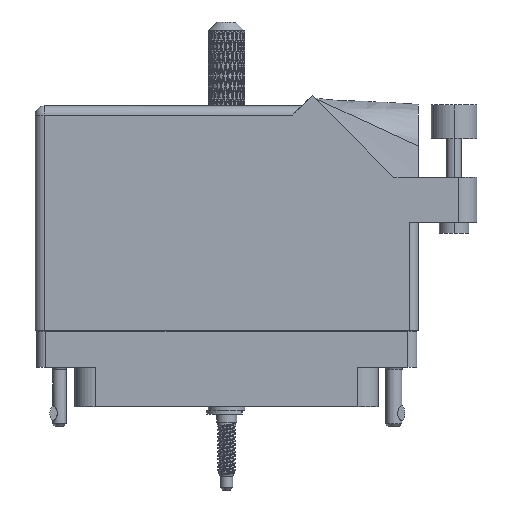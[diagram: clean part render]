
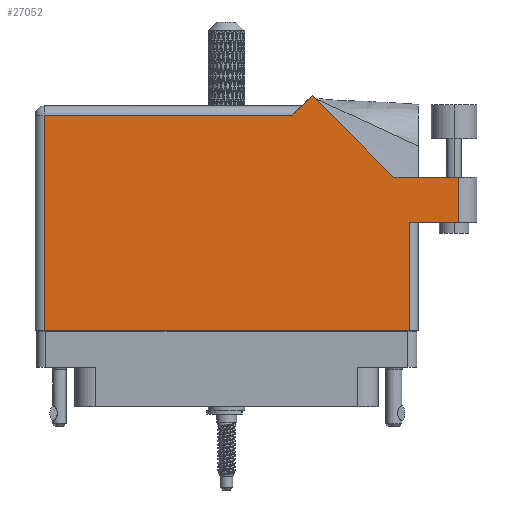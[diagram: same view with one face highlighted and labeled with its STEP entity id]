
A CAD part, front view. The second image highlights one B-rep face of the part: STEP entity #27052.
In plain terms, the highlighted face is planar.
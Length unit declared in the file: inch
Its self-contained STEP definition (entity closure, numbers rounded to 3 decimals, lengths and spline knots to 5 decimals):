
#1107 = CARTESIAN_POINT ( 'NONE',  ( 1.706, 0.944, 0.455 ) ) ;
#1807 = LINE ( 'NONE', #1107, #78496 ) ;
#3629 = VERTEX_POINT ( 'NONE', #45650 ) ;
#8971 = CARTESIAN_POINT ( 'NONE',  ( -1.244, -0.1, 0.455 ) ) ;
#10130 = DIRECTION ( 'NONE',  ( 1., 0., 0. ) ) ;
#15489 = PLANE ( 'NONE',  #107749 ) ;
#17531 = CARTESIAN_POINT ( 'NONE',  ( 1.14042, 0.944, 0.455 ) ) ;
#17821 = VERTEX_POINT ( 'NONE', #45904 ) ;
#18321 = VERTEX_POINT ( 'NONE', #92838 ) ;
#19076 = CARTESIAN_POINT ( 'NONE',  ( 0.513, 1.43, 0.455 ) ) ;
#19303 = CARTESIAN_POINT ( 'NONE',  ( -1.244, -0.1, 0.455 ) ) ;
#20014 = ORIENTED_EDGE ( 'NONE', *, *, #60571, .T. ) ;
#25834 = VECTOR ( 'NONE', #10130, 39.37008 ) ;
#27052 = ADVANCED_FACE ( 'NONE', ( #53091 ), #15489, .F. ) ;
#29794 = LINE ( 'NONE', #17531, #75566 ) ;
#30705 = VECTOR ( 'NONE', #89515, 39.37008 ) ;
#34439 = CARTESIAN_POINT ( 'NONE',  ( -1.306, 1.43, 0.455 ) ) ;
#35619 = CARTESIAN_POINT ( 'NONE',  ( 1.581, 0.944, 0.455 ) ) ;
#37146 = VERTEX_POINT ( 'NONE', #19303 ) ;
#37289 = DIRECTION ( 'NONE',  ( 1., 0., 0. ) ) ;
#37291 = DIRECTION ( 'NONE',  ( -0.707, 0.707, 0. ) ) ;
#38185 = ORIENTED_EDGE ( 'NONE', *, *, #101634, .T. ) ;
#40395 = CARTESIAN_POINT ( 'NONE',  ( 1.244, 0.637, 0.455 ) ) ;
#41104 = ORIENTED_EDGE ( 'NONE', *, *, #90923, .T. ) ;
#44049 = CARTESIAN_POINT ( 'NONE',  ( 1.581, 0.637, 0.455 ) ) ;
#45650 = CARTESIAN_POINT ( 'NONE',  ( 0.58371, 1.50071, 0.455 ) ) ;
#45701 = ORIENTED_EDGE ( 'NONE', *, *, #86420, .T. ) ;
#45733 = VECTOR ( 'NONE', #76660, 39.37008 ) ;
#45904 = CARTESIAN_POINT ( 'NONE',  ( 1.244, 0.637, 0.455 ) ) ;
#47489 = DIRECTION ( 'NONE',  ( -0.707, -0.707, 0. ) ) ;
#48413 = VECTOR ( 'NONE', #47489, 39.37008 ) ;
#49285 = VERTEX_POINT ( 'NONE', #35619 ) ;
#50863 = LINE ( 'NONE', #113680, #25834 ) ;
#53091 = FACE_OUTER_BOUND ( 'NONE', #87425, .T. ) ;
#54775 = CARTESIAN_POINT ( 'NONE',  ( 1.14042, 0.944, 0.455 ) ) ;
#56794 = LINE ( 'NONE', #81420, #117391 ) ;
#60571 = EDGE_CURVE ( 'NONE', #18321, #94752, #56794, .T. ) ;
#63276 = DIRECTION ( 'NONE',  ( -1., 0., 0. ) ) ;
#63346 = EDGE_CURVE ( 'NONE', #49285, #69453, #1807, .T. ) ;
#67115 = DIRECTION ( 'NONE',  ( -1., 0., 0. ) ) ;
#69453 = VERTEX_POINT ( 'NONE', #54775 ) ;
#70926 = LINE ( 'NONE', #111983, #112257 ) ;
#71590 = EDGE_CURVE ( 'NONE', #37146, #112481, #70926, .T. ) ;
#75566 = VECTOR ( 'NONE', #37291, 39.37008 ) ;
#76660 = DIRECTION ( 'NONE',  ( 0., 1., 0. ) ) ;
#76928 = CARTESIAN_POINT ( 'NONE',  ( -1.244, 1.368, 0.455 ) ) ;
#78496 = VECTOR ( 'NONE', #67115, 39.37008 ) ;
#79142 = ORIENTED_EDGE ( 'NONE', *, *, #71590, .T. ) ;
#79615 = CARTESIAN_POINT ( 'NONE',  ( 1.581, 0.944, 0.455 ) ) ;
#81420 = CARTESIAN_POINT ( 'NONE',  ( -1.306, 1.368, 0.455 ) ) ;
#85393 = VERTEX_POINT ( 'NONE', #44049 ) ;
#86323 = ORIENTED_EDGE ( 'NONE', *, *, #115224, .T. ) ;
#86420 = EDGE_CURVE ( 'NONE', #94752, #37146, #104943, .T. ) ;
#87425 = EDGE_LOOP ( 'NONE', ( #89865, #38185, #119226, #41104, #108203, #20014, #45701, #79142, #86323 ) ) ;
#88471 = EDGE_CURVE ( 'NONE', #3629, #18321, #114900, .T. ) ;
#88714 = VECTOR ( 'NONE', #103463, 39.37008 ) ;
#89515 = DIRECTION ( 'NONE',  ( 0., 1., 0. ) ) ;
#89865 = ORIENTED_EDGE ( 'NONE', *, *, #98420, .T. ) ;
#90923 = EDGE_CURVE ( 'NONE', #69453, #3629, #29794, .T. ) ;
#90951 = DIRECTION ( 'NONE',  ( -1., 0., 0. ) ) ;
#92838 = CARTESIAN_POINT ( 'NONE',  ( 0.451, 1.368, 0.455 ) ) ;
#94752 = VERTEX_POINT ( 'NONE', #76928 ) ;
#98420 = EDGE_CURVE ( 'NONE', #17821, #85393, #50863, .T. ) ;
#100476 = DIRECTION ( 'NONE',  ( 0., 0., -1. ) ) ;
#101634 = EDGE_CURVE ( 'NONE', #85393, #49285, #106021, .T. ) ;
#102345 = CARTESIAN_POINT ( 'NONE',  ( 1.244, -0.1, 0.455 ) ) ;
#103463 = DIRECTION ( 'NONE',  ( 0., -1., 0. ) ) ;
#104943 = LINE ( 'NONE', #8971, #88714 ) ;
#106021 = LINE ( 'NONE', #79615, #30705 ) ;
#107749 = AXIS2_PLACEMENT_3D ( 'NONE', #34439, #100476, #63276 ) ;
#108203 = ORIENTED_EDGE ( 'NONE', *, *, #88471, .T. ) ;
#111983 = CARTESIAN_POINT ( 'NONE',  ( -1.306, -0.1, 0.455 ) ) ;
#112257 = VECTOR ( 'NONE', #37289, 39.37008 ) ;
#112481 = VERTEX_POINT ( 'NONE', #102345 ) ;
#113680 = CARTESIAN_POINT ( 'NONE',  ( 1.306, 0.637, 0.455 ) ) ;
#114900 = LINE ( 'NONE', #19076, #48413 ) ;
#115224 = EDGE_CURVE ( 'NONE', #112481, #17821, #121090, .T. ) ;
#117391 = VECTOR ( 'NONE', #90951, 39.37008 ) ;
#119226 = ORIENTED_EDGE ( 'NONE', *, *, #63346, .T. ) ;
#121090 = LINE ( 'NONE', #40395, #45733 ) ;
